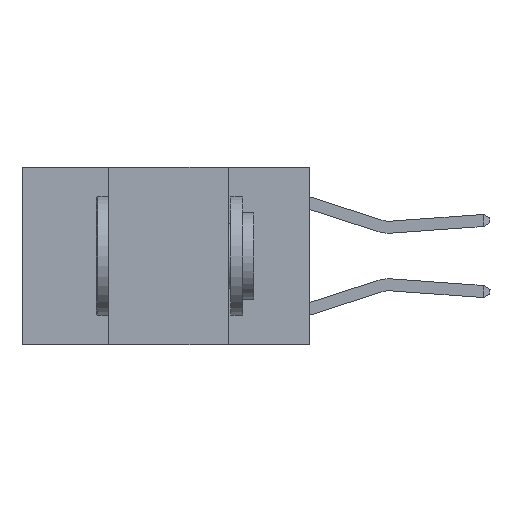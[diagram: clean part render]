
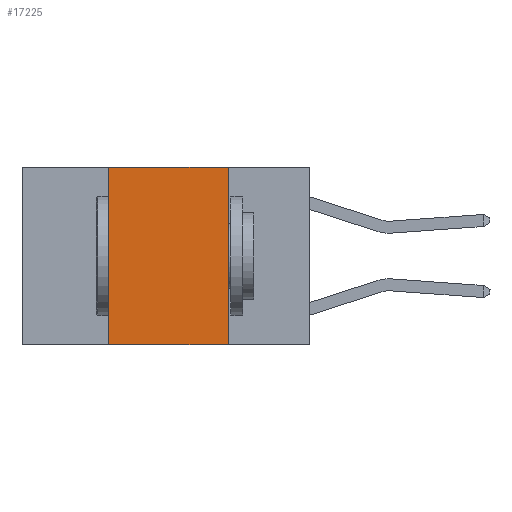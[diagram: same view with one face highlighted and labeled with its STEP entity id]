
A CAD part, left-side view. The second image highlights one B-rep face of the part: STEP entity #17225.
In plain terms, the highlighted planar face has unit normal (-1, 0, 0).
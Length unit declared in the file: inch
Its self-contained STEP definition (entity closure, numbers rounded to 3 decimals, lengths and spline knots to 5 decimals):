
#216 = CARTESIAN_POINT ( 'NONE',  ( 0., 0.6, -0.37 ) ) ;
#320 = DIRECTION ( 'NONE',  ( 0., 0., -1. ) ) ;
#974 = ORIENTED_EDGE ( 'NONE', *, *, #12430, .F. ) ;
#1219 = CARTESIAN_POINT ( 'NONE',  ( 0., 0.42, -0.37 ) ) ;
#1644 = CARTESIAN_POINT ( 'NONE',  ( 0., 0.17, -0.37 ) ) ;
#1726 = VECTOR ( 'NONE', #17723, 39.37008 ) ;
#1938 = CARTESIAN_POINT ( 'NONE',  ( 0., 0.17, 0. ) ) ;
#2016 = CARTESIAN_POINT ( 'NONE',  ( 0., 0.17, 0. ) ) ;
#2096 = DIRECTION ( 'NONE',  ( 1., 0., 0. ) ) ;
#3233 = CARTESIAN_POINT ( 'NONE',  ( 0., 0.42, 0. ) ) ;
#3277 = LINE ( 'NONE', #1938, #1726 ) ;
#4671 = VECTOR ( 'NONE', #20412, 39.37008 ) ;
#4694 = LINE ( 'NONE', #3233, #4671 ) ;
#5001 = FACE_OUTER_BOUND ( 'NONE', #15672, .T. ) ;
#6360 = LINE ( 'NONE', #216, #18228 ) ;
#6512 = VERTEX_POINT ( 'NONE', #1644 ) ;
#7765 = DIRECTION ( 'NONE',  ( 0., -1., 0. ) ) ;
#7805 = ORIENTED_EDGE ( 'NONE', *, *, #10310, .F. ) ;
#8677 = ORIENTED_EDGE ( 'NONE', *, *, #11555, .T. ) ;
#9961 = PLANE ( 'NONE',  #13389 ) ;
#10310 = EDGE_CURVE ( 'NONE', #17902, #17056, #4694, .T. ) ;
#11555 = EDGE_CURVE ( 'NONE', #17902, #6512, #6360, .T. ) ;
#12430 = EDGE_CURVE ( 'NONE', #17056, #13691, #15412, .T. ) ;
#13071 = EDGE_CURVE ( 'NONE', #13691, #6512, #3277, .T. ) ;
#13389 = AXIS2_PLACEMENT_3D ( 'NONE', #17671, #2096, #320 ) ;
#13691 = VERTEX_POINT ( 'NONE', #2016 ) ;
#14306 = VECTOR ( 'NONE', #7765, 39.37008 ) ;
#15412 = LINE ( 'NONE', #18506, #14306 ) ;
#15630 = CARTESIAN_POINT ( 'NONE',  ( 0., 0.42, 0. ) ) ;
#15672 = EDGE_LOOP ( 'NONE', ( #18477, #974, #7805, #8677 ) ) ;
#17056 = VERTEX_POINT ( 'NONE', #15630 ) ;
#17181 = DIRECTION ( 'NONE',  ( 0., -1., 0. ) ) ;
#17225 = ADVANCED_FACE ( 'NONE', ( #5001 ), #9961, .F. ) ;
#17671 = CARTESIAN_POINT ( 'NONE',  ( 0., 0.6, 0. ) ) ;
#17723 = DIRECTION ( 'NONE',  ( 0., 0., -1. ) ) ;
#17902 = VERTEX_POINT ( 'NONE', #1219 ) ;
#18228 = VECTOR ( 'NONE', #17181, 39.37008 ) ;
#18477 = ORIENTED_EDGE ( 'NONE', *, *, #13071, .F. ) ;
#18506 = CARTESIAN_POINT ( 'NONE',  ( 0., 0.6, 0. ) ) ;
#20412 = DIRECTION ( 'NONE',  ( 0., 0., 1. ) ) ;
